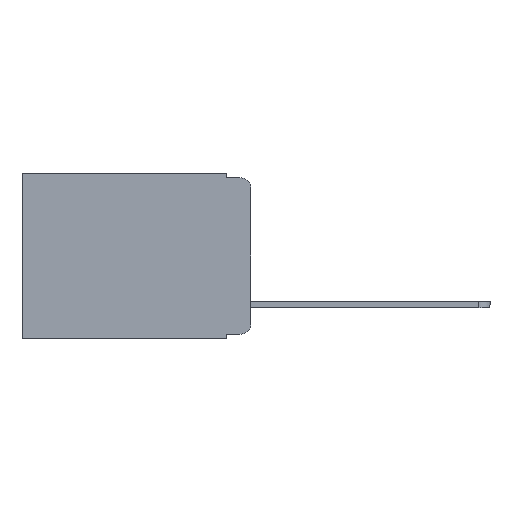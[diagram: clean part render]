
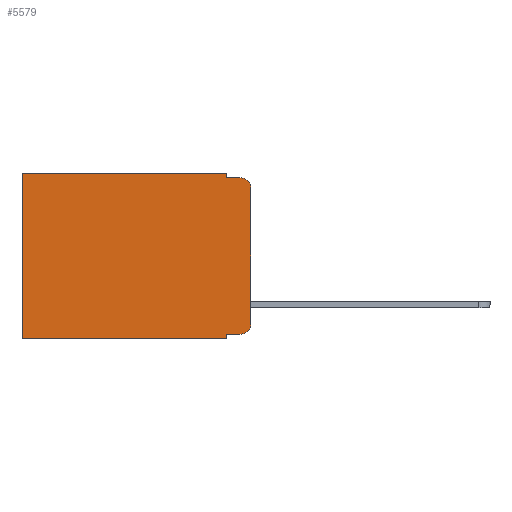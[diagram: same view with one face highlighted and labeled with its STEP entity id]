
A CAD part, left-side view. The second image highlights one B-rep face of the part: STEP entity #5579.
In plain terms, the highlighted planar face has unit normal (-1, 0, 0).
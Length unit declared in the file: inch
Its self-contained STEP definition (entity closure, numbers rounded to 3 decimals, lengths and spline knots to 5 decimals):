
#122 = DIRECTION ( 'NONE',  ( 0., -1., 0. ) ) ;
#269 = EDGE_CURVE ( 'NONE', #1558, #10609, #10698, .T. ) ;
#393 = ORIENTED_EDGE ( 'NONE', *, *, #10352, .F. ) ;
#512 = AXIS2_PLACEMENT_3D ( 'NONE', #6015, #1889, #6156 ) ;
#796 = CARTESIAN_POINT ( 'NONE',  ( 0.298, 0.02, -0.03 ) ) ;
#861 = DIRECTION ( 'NONE',  ( 0., 1., 0. ) ) ;
#929 = CARTESIAN_POINT ( 'NONE',  ( 0.298, 0.051, 0. ) ) ;
#1234 = ORIENTED_EDGE ( 'NONE', *, *, #12045, .T. ) ;
#1455 = EDGE_CURVE ( 'NONE', #10285, #1558, #3035, .T. ) ;
#1558 = VERTEX_POINT ( 'NONE', #8692 ) ;
#1697 = VECTOR ( 'NONE', #1861, 39.37008 ) ;
#1861 = DIRECTION ( 'NONE',  ( 0., 0., -1. ) ) ;
#1889 = DIRECTION ( 'NONE',  ( -1., 0., 0. ) ) ;
#1912 = DIRECTION ( 'NONE',  ( 0., 0., -1. ) ) ;
#2512 = CARTESIAN_POINT ( 'NONE',  ( 0.298, 0.473, -0.343 ) ) ;
#2710 = DIRECTION ( 'NONE',  ( 0., 0., -1. ) ) ;
#2749 = VERTEX_POINT ( 'NONE', #2512 ) ;
#2770 = LINE ( 'NONE', #12428, #1697 ) ;
#2849 = VERTEX_POINT ( 'NONE', #7305 ) ;
#3010 = EDGE_CURVE ( 'NONE', #7088, #2849, #2770, .T. ) ;
#3035 = LINE ( 'NONE', #12470, #12643 ) ;
#3039 = DIRECTION ( 'NONE',  ( 0., 1., 0. ) ) ;
#3714 = ORIENTED_EDGE ( 'NONE', *, *, #10876, .T. ) ;
#3734 = FACE_OUTER_BOUND ( 'NONE', #5618, .T. ) ;
#4106 = LINE ( 'NONE', #12230, #11227 ) ;
#4659 = LINE ( 'NONE', #7821, #8030 ) ;
#4802 = DIRECTION ( 'NONE',  ( 0., 0., -1. ) ) ;
#4940 = PLANE ( 'NONE',  #8039 ) ;
#5052 = CARTESIAN_POINT ( 'NONE',  ( 0.298, 0.473, 0. ) ) ;
#5249 = DIRECTION ( 'NONE',  ( 0., -1., 0. ) ) ;
#5285 = CARTESIAN_POINT ( 'NONE',  ( 0.298, 0.051, -0.333 ) ) ;
#5426 = CARTESIAN_POINT ( 'NONE',  ( 0.298, 0.051, -0.01 ) ) ;
#5498 = ORIENTED_EDGE ( 'NONE', *, *, #3010, .F. ) ;
#5579 = ADVANCED_FACE ( 'NONE', ( #3734 ), #4940, .F. ) ;
#5618 = EDGE_LOOP ( 'NONE', ( #7262, #5795, #8815, #13113, #6466, #1234, #393, #5498, #3714, #9496 ) ) ;
#5795 = ORIENTED_EDGE ( 'NONE', *, *, #7327, .T. ) ;
#5975 = CARTESIAN_POINT ( 'NONE',  ( 0.298, 0.473, 0. ) ) ;
#6015 = CARTESIAN_POINT ( 'NONE',  ( 0.298, 0.02, -0.313 ) ) ;
#6047 = AXIS2_PLACEMENT_3D ( 'NONE', #796, #10565, #12633 ) ;
#6156 = DIRECTION ( 'NONE',  ( 0., 0., -1. ) ) ;
#6348 = VECTOR ( 'NONE', #5249, 39.37008 ) ;
#6466 = ORIENTED_EDGE ( 'NONE', *, *, #7607, .T. ) ;
#6556 = LINE ( 'NONE', #11814, #6348 ) ;
#7088 = VERTEX_POINT ( 'NONE', #5285 ) ;
#7262 = ORIENTED_EDGE ( 'NONE', *, *, #12531, .F. ) ;
#7305 = CARTESIAN_POINT ( 'NONE',  ( 0.298, 0.051, -0.343 ) ) ;
#7327 = EDGE_CURVE ( 'NONE', #8493, #10609, #10279, .T. ) ;
#7607 = EDGE_CURVE ( 'NONE', #10285, #13305, #4659, .T. ) ;
#7821 = CARTESIAN_POINT ( 'NONE',  ( 0.298, 0., 0. ) ) ;
#8030 = VECTOR ( 'NONE', #3039, 39.37008 ) ;
#8039 = AXIS2_PLACEMENT_3D ( 'NONE', #12274, #13248, #4802 ) ;
#8071 = DIRECTION ( 'NONE',  ( 0., 0., -1. ) ) ;
#8493 = VERTEX_POINT ( 'NONE', #11002 ) ;
#8632 = EDGE_CURVE ( 'NONE', #9467, #9504, #8718, .T. ) ;
#8682 = CARTESIAN_POINT ( 'NONE',  ( 0.298, 0.02, -0.333 ) ) ;
#8692 = CARTESIAN_POINT ( 'NONE',  ( 0.298, 0.051, -0.01 ) ) ;
#8718 = CIRCLE ( 'NONE', #512, 0.02 ) ;
#8815 = ORIENTED_EDGE ( 'NONE', *, *, #269, .F. ) ;
#9292 = CARTESIAN_POINT ( 'NONE',  ( 0.298, 0., -0.343 ) ) ;
#9342 = LINE ( 'NONE', #5052, #11643 ) ;
#9430 = LINE ( 'NONE', #9292, #10051 ) ;
#9467 = VERTEX_POINT ( 'NONE', #8682 ) ;
#9496 = ORIENTED_EDGE ( 'NONE', *, *, #8632, .T. ) ;
#9504 = VERTEX_POINT ( 'NONE', #10639 ) ;
#10050 = VECTOR ( 'NONE', #122, 39.37008 ) ;
#10051 = VECTOR ( 'NONE', #861, 39.37008 ) ;
#10279 = CIRCLE ( 'NONE', #6047, 0.02 ) ;
#10285 = VERTEX_POINT ( 'NONE', #929 ) ;
#10352 = EDGE_CURVE ( 'NONE', #2849, #2749, #9430, .T. ) ;
#10565 = DIRECTION ( 'NONE',  ( -1., 0., 0. ) ) ;
#10609 = VERTEX_POINT ( 'NONE', #12037 ) ;
#10639 = CARTESIAN_POINT ( 'NONE',  ( 0.298, 0., -0.313 ) ) ;
#10698 = LINE ( 'NONE', #5426, #10050 ) ;
#10876 = EDGE_CURVE ( 'NONE', #7088, #9467, #6556, .T. ) ;
#11002 = CARTESIAN_POINT ( 'NONE',  ( 0.298, 0., -0.03 ) ) ;
#11227 = VECTOR ( 'NONE', #2710, 39.37008 ) ;
#11643 = VECTOR ( 'NONE', #8071, 39.37008 ) ;
#11814 = CARTESIAN_POINT ( 'NONE',  ( 0.298, 0.051, -0.333 ) ) ;
#12037 = CARTESIAN_POINT ( 'NONE',  ( 0.298, 0.02, -0.01 ) ) ;
#12045 = EDGE_CURVE ( 'NONE', #13305, #2749, #9342, .T. ) ;
#12230 = CARTESIAN_POINT ( 'NONE',  ( 0.298, 0., 0. ) ) ;
#12274 = CARTESIAN_POINT ( 'NONE',  ( 0.298, 0., 0. ) ) ;
#12428 = CARTESIAN_POINT ( 'NONE',  ( 0.298, 0.051, 0. ) ) ;
#12470 = CARTESIAN_POINT ( 'NONE',  ( 0.298, 0.051, 0. ) ) ;
#12531 = EDGE_CURVE ( 'NONE', #8493, #9504, #4106, .T. ) ;
#12633 = DIRECTION ( 'NONE',  ( 0., 0., -1. ) ) ;
#12643 = VECTOR ( 'NONE', #1912, 39.37008 ) ;
#13113 = ORIENTED_EDGE ( 'NONE', *, *, #1455, .F. ) ;
#13248 = DIRECTION ( 'NONE',  ( 1., 0., 0. ) ) ;
#13305 = VERTEX_POINT ( 'NONE', #5975 ) ;
